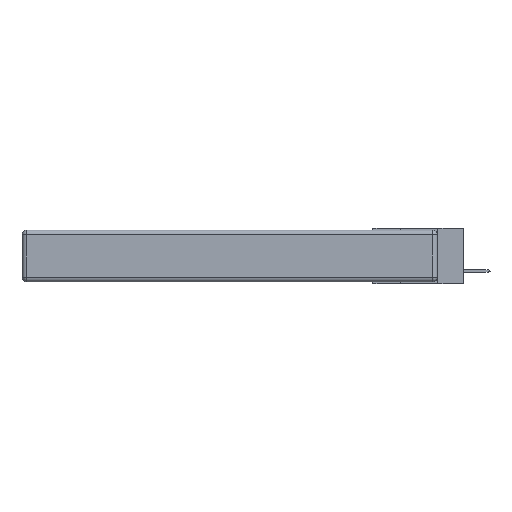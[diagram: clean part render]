
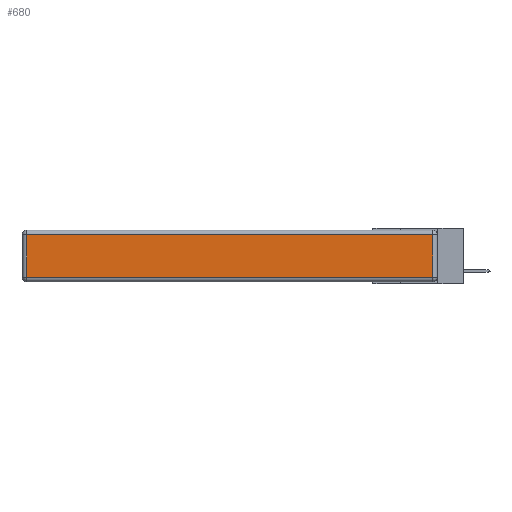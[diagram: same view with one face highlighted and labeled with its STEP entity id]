
A CAD part, left-side view. The second image highlights one B-rep face of the part: STEP entity #680.
In plain terms, the highlighted planar face has unit normal (-1, 0, 0).
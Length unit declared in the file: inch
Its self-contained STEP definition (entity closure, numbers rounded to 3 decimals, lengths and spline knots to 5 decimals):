
#680 = ADVANCED_FACE ( 'NONE', ( #6206 ), #5316, .T. ) ;
#716 = VECTOR ( 'NONE', #4917, 39.37008 ) ;
#899 = CARTESIAN_POINT ( 'NONE',  ( 0., 2.75, -0.03 ) ) ;
#1012 = CARTESIAN_POINT ( 'NONE',  ( 0., 0., -0.313 ) ) ;
#1981 = CARTESIAN_POINT ( 'NONE',  ( 0., 0.03, -0.313 ) ) ;
#2146 = CARTESIAN_POINT ( 'NONE',  ( 0., 2.72, -0.03 ) ) ;
#2288 = DIRECTION ( 'NONE',  ( 0., 0., 1. ) ) ;
#2454 = CARTESIAN_POINT ( 'NONE',  ( 0., 2.72, -0.343 ) ) ;
#2864 = CARTESIAN_POINT ( 'NONE',  ( 0., 0.03, -0.343 ) ) ;
#2903 = DIRECTION ( 'NONE',  ( 0., -1., 0. ) ) ;
#3149 = ORIENTED_EDGE ( 'NONE', *, *, #5477, .T. ) ;
#3170 = LINE ( 'NONE', #1012, #7729 ) ;
#3412 = ORIENTED_EDGE ( 'NONE', *, *, #7358, .T. ) ;
#3435 = DIRECTION ( 'NONE',  ( 0., 0., -1. ) ) ;
#3703 = CARTESIAN_POINT ( 'NONE',  ( 0., 2.72, -0.313 ) ) ;
#4045 = CARTESIAN_POINT ( 'NONE',  ( 0., 0., -0.343 ) ) ;
#4917 = DIRECTION ( 'NONE',  ( 0., 1., 0. ) ) ;
#5011 = LINE ( 'NONE', #899, #716 ) ;
#5143 = EDGE_CURVE ( 'NONE', #10396, #12634, #5011, .T. ) ;
#5316 = PLANE ( 'NONE',  #7034 ) ;
#5477 = EDGE_CURVE ( 'NONE', #12326, #9425, #3170, .T. ) ;
#5684 = CARTESIAN_POINT ( 'NONE',  ( 0., 0.03, -0.03 ) ) ;
#5799 = DIRECTION ( 'NONE',  ( 0., 0., 1. ) ) ;
#6135 = EDGE_CURVE ( 'NONE', #12634, #12326, #7701, .T. ) ;
#6206 = FACE_OUTER_BOUND ( 'NONE', #12276, .T. ) ;
#6298 = LINE ( 'NONE', #2864, #6751 ) ;
#6751 = VECTOR ( 'NONE', #5799, 39.37008 ) ;
#7034 = AXIS2_PLACEMENT_3D ( 'NONE', #4045, #7189, #2288 ) ;
#7189 = DIRECTION ( 'NONE',  ( -1., 0., 0. ) ) ;
#7358 = EDGE_CURVE ( 'NONE', #9425, #10396, #6298, .T. ) ;
#7701 = LINE ( 'NONE', #2454, #12307 ) ;
#7729 = VECTOR ( 'NONE', #2903, 39.37008 ) ;
#8471 = ORIENTED_EDGE ( 'NONE', *, *, #5143, .T. ) ;
#9227 = ORIENTED_EDGE ( 'NONE', *, *, #6135, .T. ) ;
#9425 = VERTEX_POINT ( 'NONE', #1981 ) ;
#10396 = VERTEX_POINT ( 'NONE', #5684 ) ;
#12276 = EDGE_LOOP ( 'NONE', ( #3149, #3412, #8471, #9227 ) ) ;
#12307 = VECTOR ( 'NONE', #3435, 39.37008 ) ;
#12326 = VERTEX_POINT ( 'NONE', #3703 ) ;
#12634 = VERTEX_POINT ( 'NONE', #2146 ) ;
